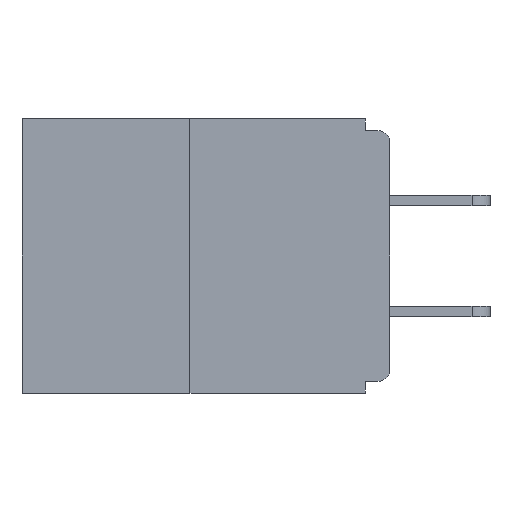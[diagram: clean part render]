
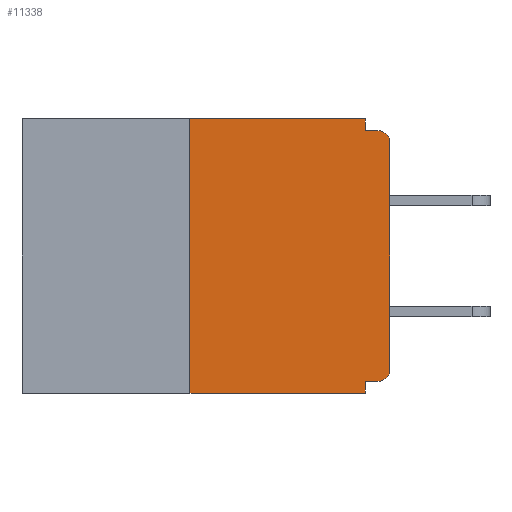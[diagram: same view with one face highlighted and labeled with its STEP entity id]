
A CAD part, left-side view. The second image highlights one B-rep face of the part: STEP entity #11338.
In plain terms, the highlighted planar face has unit normal (-1, 0, 0).
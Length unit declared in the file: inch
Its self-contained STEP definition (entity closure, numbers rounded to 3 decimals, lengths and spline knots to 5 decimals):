
#105 = CARTESIAN_POINT ( 'NONE',  ( 0., 0.25, -0.343 ) ) ;
#353 = CARTESIAN_POINT ( 'NONE',  ( 0., 0.015, -0.015 ) ) ;
#537 = DIRECTION ( 'NONE',  ( 0., 0., 1. ) ) ;
#657 = CARTESIAN_POINT ( 'NONE',  ( 0., 0., 0. ) ) ;
#780 = PLANE ( 'NONE',  #1648 ) ;
#1304 = DIRECTION ( 'NONE',  ( 0., 0., 1. ) ) ;
#1365 = ORIENTED_EDGE ( 'NONE', *, *, #5357, .F. ) ;
#1648 = AXIS2_PLACEMENT_3D ( 'NONE', #6145, #1888, #11577 ) ;
#1888 = DIRECTION ( 'NONE',  ( 1., 0., 0. ) ) ;
#2030 = DIRECTION ( 'NONE',  ( -1., 0., 0. ) ) ;
#2123 = LINE ( 'NONE', #3092, #13967 ) ;
#2409 = ORIENTED_EDGE ( 'NONE', *, *, #11320, .T. ) ;
#2472 = VERTEX_POINT ( 'NONE', #7060 ) ;
#3092 = CARTESIAN_POINT ( 'NONE',  ( 0., 0., -0.328 ) ) ;
#3369 = EDGE_CURVE ( 'NONE', #16132, #15759, #10171, .T. ) ;
#3654 = VECTOR ( 'NONE', #12019, 39.37008 ) ;
#3657 = ORIENTED_EDGE ( 'NONE', *, *, #3369, .T. ) ;
#3812 = VERTEX_POINT ( 'NONE', #12029 ) ;
#3929 = ORIENTED_EDGE ( 'NONE', *, *, #6058, .F. ) ;
#3997 = DIRECTION ( 'NONE',  ( 0., 0., -1. ) ) ;
#4103 = CARTESIAN_POINT ( 'NONE',  ( 0., 0.031, -0.015 ) ) ;
#4200 = LINE ( 'NONE', #14046, #16176 ) ;
#4246 = ORIENTED_EDGE ( 'NONE', *, *, #11855, .T. ) ;
#4481 = DIRECTION ( 'NONE',  ( 0., 0., -1. ) ) ;
#4541 = CARTESIAN_POINT ( 'NONE',  ( 0., 0.031, -0.343 ) ) ;
#4699 = AXIS2_PLACEMENT_3D ( 'NONE', #15141, #12404, #3997 ) ;
#4792 = VECTOR ( 'NONE', #13061, 39.37008 ) ;
#4890 = VECTOR ( 'NONE', #1304, 39.37008 ) ;
#5167 = LINE ( 'NONE', #7793, #3654 ) ;
#5218 = LINE ( 'NONE', #6965, #6284 ) ;
#5229 = VERTEX_POINT ( 'NONE', #4103 ) ;
#5357 = EDGE_CURVE ( 'NONE', #17480, #2472, #16220, .T. ) ;
#5624 = VERTEX_POINT ( 'NONE', #353 ) ;
#5870 = CARTESIAN_POINT ( 'NONE',  ( 0., 0., -0.313 ) ) ;
#6058 = EDGE_CURVE ( 'NONE', #3812, #7069, #17492, .T. ) ;
#6145 = CARTESIAN_POINT ( 'NONE',  ( 0., 0.46, 0. ) ) ;
#6284 = VECTOR ( 'NONE', #9555, 39.37008 ) ;
#6729 = CARTESIAN_POINT ( 'NONE',  ( 0., 0.25, 0. ) ) ;
#6965 = CARTESIAN_POINT ( 'NONE',  ( 0., 0.031, 0. ) ) ;
#7060 = CARTESIAN_POINT ( 'NONE',  ( 0., 0.25, 0. ) ) ;
#7069 = VERTEX_POINT ( 'NONE', #11946 ) ;
#7793 = CARTESIAN_POINT ( 'NONE',  ( 0., 0.46, 0. ) ) ;
#8401 = CARTESIAN_POINT ( 'NONE',  ( 0., 0.031, 0. ) ) ;
#8429 = FACE_OUTER_BOUND ( 'NONE', #10724, .T. ) ;
#8585 = DIRECTION ( 'NONE',  ( 0., 1., 0. ) ) ;
#8594 = VECTOR ( 'NONE', #4481, 39.37008 ) ;
#8748 = EDGE_CURVE ( 'NONE', #5229, #5624, #11295, .T. ) ;
#9345 = ORIENTED_EDGE ( 'NONE', *, *, #13654, .T. ) ;
#9470 = EDGE_CURVE ( 'NONE', #17701, #5229, #5218, .T. ) ;
#9555 = DIRECTION ( 'NONE',  ( 0., 0., -1. ) ) ;
#10021 = ORIENTED_EDGE ( 'NONE', *, *, #11124, .F. ) ;
#10075 = DIRECTION ( 'NONE',  ( 0., -1., 0. ) ) ;
#10171 = CIRCLE ( 'NONE', #4699, 0.015 ) ;
#10332 = CARTESIAN_POINT ( 'NONE',  ( 0., 0.015, -0.03 ) ) ;
#10657 = VECTOR ( 'NONE', #537, 39.37008 ) ;
#10724 = EDGE_LOOP ( 'NONE', ( #17396, #1365, #9345, #3929, #10021, #3657, #2409, #4246, #14991, #14967 ) ) ;
#10766 = CARTESIAN_POINT ( 'NONE',  ( 0., 0.015, -0.328 ) ) ;
#10830 = EDGE_CURVE ( 'NONE', #2472, #17701, #5167, .T. ) ;
#11124 = EDGE_CURVE ( 'NONE', #16132, #3812, #2123, .T. ) ;
#11295 = LINE ( 'NONE', #17067, #4792 ) ;
#11320 = EDGE_CURVE ( 'NONE', #15759, #14382, #12704, .T. ) ;
#11338 = ADVANCED_FACE ( 'NONE', ( #8429 ), #780, .F. ) ;
#11577 = DIRECTION ( 'NONE',  ( 0., 0., -1. ) ) ;
#11721 = DIRECTION ( 'NONE',  ( 0., 0., -1. ) ) ;
#11855 = EDGE_CURVE ( 'NONE', #14382, #5624, #13106, .T. ) ;
#11946 = CARTESIAN_POINT ( 'NONE',  ( 0., 0.031, -0.343 ) ) ;
#12019 = DIRECTION ( 'NONE',  ( 0., -1., 0. ) ) ;
#12029 = CARTESIAN_POINT ( 'NONE',  ( 0., 0.031, -0.328 ) ) ;
#12404 = DIRECTION ( 'NONE',  ( -1., 0., 0. ) ) ;
#12704 = LINE ( 'NONE', #657, #10657 ) ;
#12864 = CARTESIAN_POINT ( 'NONE',  ( 0., 0., -0.03 ) ) ;
#13061 = DIRECTION ( 'NONE',  ( 0., -1., 0. ) ) ;
#13106 = CIRCLE ( 'NONE', #17479, 0.015 ) ;
#13654 = EDGE_CURVE ( 'NONE', #17480, #7069, #4200, .T. ) ;
#13967 = VECTOR ( 'NONE', #8585, 39.37008 ) ;
#14046 = CARTESIAN_POINT ( 'NONE',  ( 0., 0.46, -0.343 ) ) ;
#14382 = VERTEX_POINT ( 'NONE', #12864 ) ;
#14967 = ORIENTED_EDGE ( 'NONE', *, *, #9470, .F. ) ;
#14991 = ORIENTED_EDGE ( 'NONE', *, *, #8748, .F. ) ;
#15141 = CARTESIAN_POINT ( 'NONE',  ( 0., 0.015, -0.313 ) ) ;
#15759 = VERTEX_POINT ( 'NONE', #5870 ) ;
#16132 = VERTEX_POINT ( 'NONE', #10766 ) ;
#16176 = VECTOR ( 'NONE', #10075, 39.37008 ) ;
#16220 = LINE ( 'NONE', #6729, #4890 ) ;
#17067 = CARTESIAN_POINT ( 'NONE',  ( 0., 0., -0.015 ) ) ;
#17396 = ORIENTED_EDGE ( 'NONE', *, *, #10830, .F. ) ;
#17479 = AXIS2_PLACEMENT_3D ( 'NONE', #10332, #2030, #11721 ) ;
#17480 = VERTEX_POINT ( 'NONE', #105 ) ;
#17492 = LINE ( 'NONE', #4541, #8594 ) ;
#17701 = VERTEX_POINT ( 'NONE', #8401 ) ;
